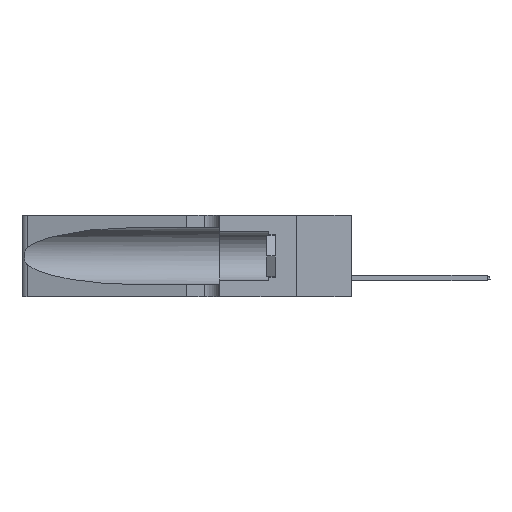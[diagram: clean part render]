
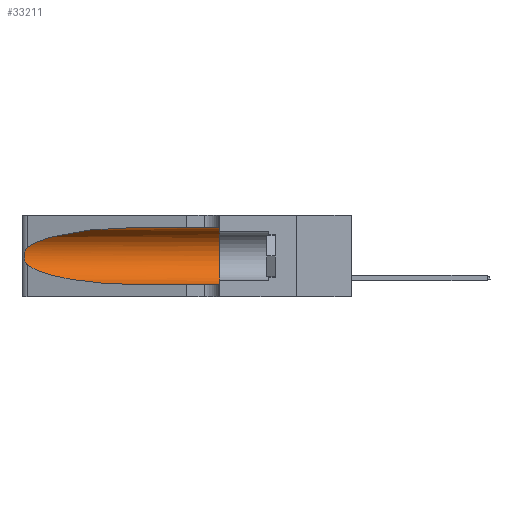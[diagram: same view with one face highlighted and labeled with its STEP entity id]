
A CAD part, left-side view. The second image highlights one B-rep face of the part: STEP entity #33211.
In plain terms, the highlighted cylindrical face has radius 3.308 mm (diameter 6.617 mm), a partial arc.
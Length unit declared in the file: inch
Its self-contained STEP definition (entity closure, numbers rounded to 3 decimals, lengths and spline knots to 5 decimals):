
#699 = CARTESIAN_POINT ( 'NONE',  ( 0.25639, 1.23184, 0.21858 ) ) ;
#844 =( BOUNDED_CURVE ( )  B_SPLINE_CURVE ( 3, ( #28350, #46144, #6914, #35526 ),
 .UNSPECIFIED., .F., .F. ) 
 B_SPLINE_CURVE_WITH_KNOTS ( ( 4, 4 ),
 ( 1.5708, 2.84003 ),
 .UNSPECIFIED. ) 
 CURVE ( )  GEOMETRIC_REPRESENTATION_ITEM ( )  RATIONAL_B_SPLINE_CURVE ( ( 1., 0.87, 0.87, 1. ) ) 
 REPRESENTATION_ITEM ( '' )  );
#1693 = CARTESIAN_POINT ( 'NONE',  ( 0.25854, 1.2359, 0.20912 ) ) ;
#1909 = VECTOR ( 'NONE', #36464, 39.37008 ) ;
#1945 = CARTESIAN_POINT ( 'NONE',  ( 0.2373, 1.15595, 0.08982 ) ) ;
#2906 = ORIENTED_EDGE ( 'NONE', *, *, #32295, .T. ) ;
#3238 = CARTESIAN_POINT ( 'NONE',  ( 0.1305, 0.35, 0.31525 ) ) ;
#3974 = CARTESIAN_POINT ( 'NONE',  ( 0.1305, 1.61858, 0.05475 ) ) ;
#3989 = CARTESIAN_POINT ( 'NONE',  ( 0.25555, 1.22993, 0.14849 ) ) ;
#4101 = DIRECTION ( 'NONE',  ( 0., -1., 0. ) ) ;
#4175 = CARTESIAN_POINT ( 'NONE',  ( 0.25487, 1.22718, 0.22369 ) ) ;
#5807 = FACE_OUTER_BOUND ( 'NONE', #34516, .T. ) ;
#6914 = CARTESIAN_POINT ( 'NONE',  ( 0.2373, 1.15595, 0.28018 ) ) ;
#7427 = CARTESIAN_POINT ( 'NONE',  ( 0.25487, 1.22718, 0.22369 ) ) ;
#7870 = CARTESIAN_POINT ( 'NONE',  ( 0.25787, 1.23484, 0.2124 ) ) ;
#8352 = CARTESIAN_POINT ( 'NONE',  ( 0.26075, 1.23896, 0.19203 ) ) ;
#8518 = CARTESIAN_POINT ( 'NONE',  ( 0.25789, 1.23486, 0.15765 ) ) ;
#8691 = AXIS2_PLACEMENT_3D ( 'NONE', #21794, #4101, #14786 ) ;
#9525 = ORIENTED_EDGE ( 'NONE', *, *, #22378, .T. ) ;
#11684 = AXIS2_PLACEMENT_3D ( 'NONE', #31947, #17735, #22200 ) ;
#11869 = CARTESIAN_POINT ( 'NONE',  ( 0.26075, 1.23896, 0.178 ) ) ;
#13083 = CARTESIAN_POINT ( 'NONE',  ( 0.1305, 0.72297, 0.31525 ) ) ;
#14599 = ORIENTED_EDGE ( 'NONE', *, *, #24858, .F. ) ;
#14786 = DIRECTION ( 'NONE',  ( 0., 0., -1. ) ) ;
#15477 = CARTESIAN_POINT ( 'NONE',  ( 0.26017, 1.23833, 0.17102 ) ) ;
#17052 = EDGE_CURVE ( 'NONE', #35445, #31300, #39383, .T. ) ;
#17735 = DIRECTION ( 'NONE',  ( 0., 1., 0. ) ) ;
#18224 = ORIENTED_EDGE ( 'NONE', *, *, #27168, .T. ) ;
#18273 = CARTESIAN_POINT ( 'NONE',  ( 0.25487, 1.22718, 0.14631 ) ) ;
#19854 = VECTOR ( 'NONE', #34056, 39.37008 ) ;
#21003 = ORIENTED_EDGE ( 'NONE', *, *, #17052, .F. ) ;
#21794 = CARTESIAN_POINT ( 'NONE',  ( 0.1305, 1.61858, 0.185 ) ) ;
#22200 = DIRECTION ( 'NONE',  ( 0., 0., 1. ) ) ;
#22378 = EDGE_CURVE ( 'NONE', #35445, #26670, #844, .T. ) ;
#24858 = EDGE_CURVE ( 'NONE', #31300, #43933, #42821, .T. ) ;
#25534 = CARTESIAN_POINT ( 'NONE',  ( 0.25487, 1.22718, 0.14631 ) ) ;
#26091 = CARTESIAN_POINT ( 'NONE',  ( 0.26018, 1.23835, 0.19895 ) ) ;
#26670 = VERTEX_POINT ( 'NONE', #7427 ) ;
#27168 = EDGE_CURVE ( 'NONE', #42926, #43933, #30303, .T. ) ;
#28350 = CARTESIAN_POINT ( 'NONE',  ( 0.1305, 0.72297, 0.31525 ) ) ;
#29877 = EDGE_CURVE ( 'NONE', #26670, #31943, #39439, .T. ) ;
#30303 = LINE ( 'NONE', #3974, #1909 ) ;
#30696 = CARTESIAN_POINT ( 'NONE',  ( 0.1305, 0.72297, 0.05475 ) ) ;
#30743 = CARTESIAN_POINT ( 'NONE',  ( 0.1305, 0.35, 0.05475 ) ) ;
#30965 = CARTESIAN_POINT ( 'NONE',  ( 0.25639, 1.23186, 0.15144 ) ) ;
#31300 = VERTEX_POINT ( 'NONE', #3238 ) ;
#31943 = VERTEX_POINT ( 'NONE', #18273 ) ;
#31947 = CARTESIAN_POINT ( 'NONE',  ( 0.1305, 0.35, 0.185 ) ) ;
#32295 = EDGE_CURVE ( 'NONE', #31943, #42926, #38052, .T. ) ;
#32626 = CARTESIAN_POINT ( 'NONE',  ( 0.25555, 1.22994, 0.2215 ) ) ;
#33178 = CARTESIAN_POINT ( 'NONE',  ( 0.25487, 1.22718, 0.14631 ) ) ;
#33211 = ADVANCED_FACE ( 'NONE', ( #5807 ), #35842, .F. ) ;
#34056 = DIRECTION ( 'NONE',  ( 0., -1., 0. ) ) ;
#34362 = CARTESIAN_POINT ( 'NONE',  ( 0.1305, 1.61858, 0.31525 ) ) ;
#34516 = EDGE_LOOP ( 'NONE', ( #9525, #35063, #2906, #18224, #14599, #21003 ) ) ;
#35063 = ORIENTED_EDGE ( 'NONE', *, *, #29877, .T. ) ;
#35445 = VERTEX_POINT ( 'NONE', #13083 ) ;
#35526 = CARTESIAN_POINT ( 'NONE',  ( 0.25487, 1.22718, 0.22369 ) ) ;
#35668 = CARTESIAN_POINT ( 'NONE',  ( 0.1305, 0.72297, 0.05475 ) ) ;
#35842 = CYLINDRICAL_SURFACE ( 'NONE', #8691, 0.13025 ) ;
#36464 = DIRECTION ( 'NONE',  ( 0., -1., 0. ) ) ;
#38052 =( BOUNDED_CURVE ( )  B_SPLINE_CURVE ( 3, ( #33178, #1945, #45710, #30696 ),
 .UNSPECIFIED., .F., .F. ) 
 B_SPLINE_CURVE_WITH_KNOTS ( ( 4, 4 ),
 ( 3.44316, 4.71239 ),
 .UNSPECIFIED. ) 
 CURVE ( )  GEOMETRIC_REPRESENTATION_ITEM ( )  RATIONAL_B_SPLINE_CURVE ( ( 1., 0.87, 0.87, 1. ) ) 
 REPRESENTATION_ITEM ( '' )  );
#39383 = LINE ( 'NONE', #34362, #19854 ) ;
#39439 = B_SPLINE_CURVE_WITH_KNOTS ( 'NONE', 3,
 ( #4175, #32626, #699, #7870, #1693, #26091, #8352, #11869, #15477, #40443, #8518, #30965, #3989, #25534 ),
 .UNSPECIFIED., .F., .F.,
 ( 4, 2, 2, 2, 2, 2, 4 ),
 ( 0., 0.00027, 0.00053, 0.00107, 0.0016, 0.00187, 0.00214 ),
 .UNSPECIFIED. ) ;
#40443 = CARTESIAN_POINT ( 'NONE',  ( 0.25856, 1.23593, 0.16098 ) ) ;
#42821 = CIRCLE ( 'NONE', #11684, 0.13025 ) ;
#42926 = VERTEX_POINT ( 'NONE', #35668 ) ;
#43933 = VERTEX_POINT ( 'NONE', #30743 ) ;
#45710 = CARTESIAN_POINT ( 'NONE',  ( 0.18966, 0.96281, 0.05475 ) ) ;
#46144 = CARTESIAN_POINT ( 'NONE',  ( 0.18966, 0.96281, 0.31525 ) ) ;
